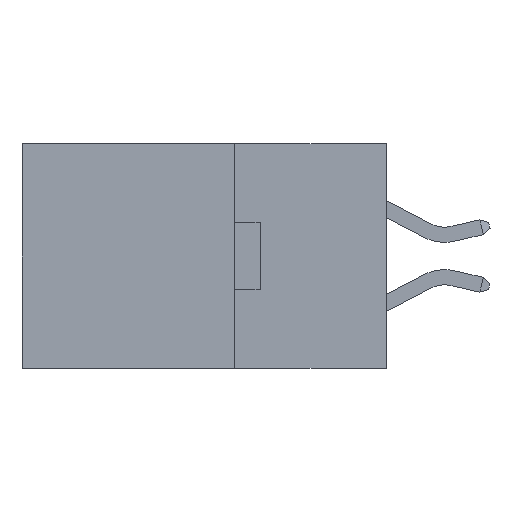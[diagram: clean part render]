
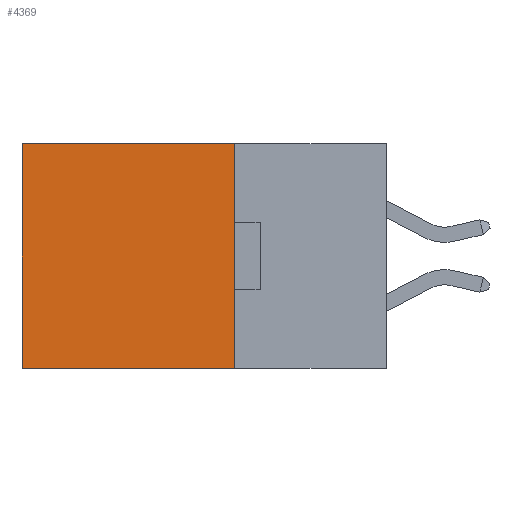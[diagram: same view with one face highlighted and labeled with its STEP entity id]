
A CAD part, left-side view. The second image highlights one B-rep face of the part: STEP entity #4369.
In plain terms, the highlighted planar face has unit normal (-1, 0, 0).
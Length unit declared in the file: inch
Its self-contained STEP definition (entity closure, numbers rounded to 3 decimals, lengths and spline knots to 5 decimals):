
#2098 = EDGE_CURVE ( 'NONE', #11747, #22398, #20240, .T. ) ;
#2567 = VERTEX_POINT ( 'NONE', #24291 ) ;
#4045 = VECTOR ( 'NONE', #12092, 39.37008 ) ;
#4369 = ADVANCED_FACE ( 'NONE', ( #20768 ), #7655, .F. ) ;
#5599 = CARTESIAN_POINT ( 'NONE',  ( 0.2615, 0.25, 0. ) ) ;
#6624 = ORIENTED_EDGE ( 'NONE', *, *, #21676, .F. ) ;
#7655 = PLANE ( 'NONE',  #25836 ) ;
#7729 = VECTOR ( 'NONE', #22680, 39.37008 ) ;
#8853 = VECTOR ( 'NONE', #14441, 39.37008 ) ;
#9208 = VERTEX_POINT ( 'NONE', #16839 ) ;
#9245 = DIRECTION ( 'NONE',  ( 0., 1., 0. ) ) ;
#9795 = DIRECTION ( 'NONE',  ( 1., 0., 0. ) ) ;
#11174 = LINE ( 'NONE', #5599, #4045 ) ;
#11747 = VERTEX_POINT ( 'NONE', #19250 ) ;
#11944 = CARTESIAN_POINT ( 'NONE',  ( 0.2615, 0.6, -0.37 ) ) ;
#12092 = DIRECTION ( 'NONE',  ( 0., 1., 0. ) ) ;
#14430 = EDGE_CURVE ( 'NONE', #2567, #11747, #11174, .T. ) ;
#14441 = DIRECTION ( 'NONE',  ( 0., 0., -1. ) ) ;
#15095 = LINE ( 'NONE', #19914, #25847 ) ;
#16293 = CARTESIAN_POINT ( 'NONE',  ( 0.2615, 0.25, -0.37 ) ) ;
#16839 = CARTESIAN_POINT ( 'NONE',  ( 0.2615, 0.25, -0.37 ) ) ;
#18678 = CARTESIAN_POINT ( 'NONE',  ( 0.2615, 0.6, -0.37 ) ) ;
#19250 = CARTESIAN_POINT ( 'NONE',  ( 0.2615, 0.6, 0. ) ) ;
#19914 = CARTESIAN_POINT ( 'NONE',  ( 0.2615, 0.25, -0.37 ) ) ;
#20240 = LINE ( 'NONE', #18678, #8853 ) ;
#20768 = FACE_OUTER_BOUND ( 'NONE', #25295, .T. ) ;
#21676 = EDGE_CURVE ( 'NONE', #2567, #9208, #24809, .T. ) ;
#21781 = ORIENTED_EDGE ( 'NONE', *, *, #23918, .F. ) ;
#22398 = VERTEX_POINT ( 'NONE', #11944 ) ;
#22622 = CARTESIAN_POINT ( 'NONE',  ( 0.2615, 0.25, -0.37 ) ) ;
#22680 = DIRECTION ( 'NONE',  ( 0., 0., -1. ) ) ;
#23918 = EDGE_CURVE ( 'NONE', #9208, #22398, #15095, .T. ) ;
#24291 = CARTESIAN_POINT ( 'NONE',  ( 0.2615, 0.25, 0. ) ) ;
#24576 = ORIENTED_EDGE ( 'NONE', *, *, #14430, .T. ) ;
#24775 = DIRECTION ( 'NONE',  ( 0., 0., -1. ) ) ;
#24809 = LINE ( 'NONE', #16293, #7729 ) ;
#25295 = EDGE_LOOP ( 'NONE', ( #27390, #21781, #6624, #24576 ) ) ;
#25836 = AXIS2_PLACEMENT_3D ( 'NONE', #22622, #9795, #24775 ) ;
#25847 = VECTOR ( 'NONE', #9245, 39.37008 ) ;
#27390 = ORIENTED_EDGE ( 'NONE', *, *, #2098, .T. ) ;
